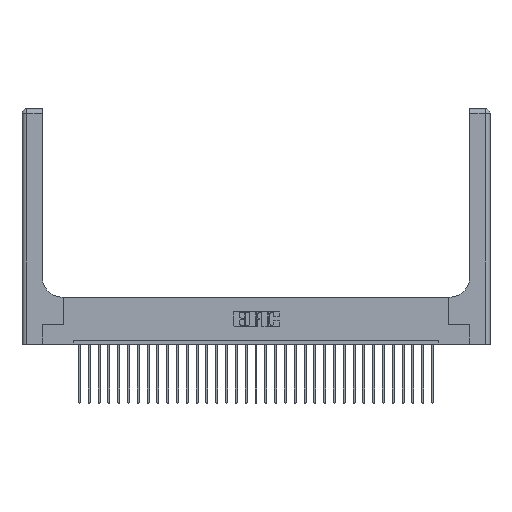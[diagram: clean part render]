
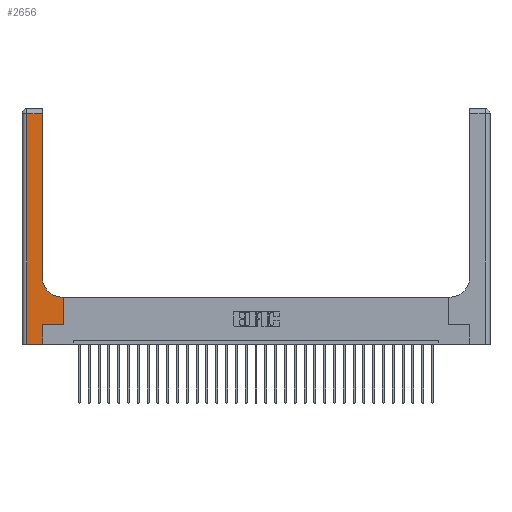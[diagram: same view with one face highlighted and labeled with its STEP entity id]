
A CAD part, top view. The second image highlights one B-rep face of the part: STEP entity #2656.
In plain terms, the highlighted planar face has unit normal (0, 0, 1).
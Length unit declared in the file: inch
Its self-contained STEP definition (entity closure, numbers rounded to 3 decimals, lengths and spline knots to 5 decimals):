
#315 = LINE ( 'NONE', #9708, #10442 ) ;
#465 = LINE ( 'NONE', #26580, #18262 ) ;
#1028 = CARTESIAN_POINT ( 'NONE',  ( 0.06, 2.94, 0.37 ) ) ;
#1530 = VERTEX_POINT ( 'NONE', #1028 ) ;
#1905 = DIRECTION ( 'NONE',  ( 1., 0., 0. ) ) ;
#2060 = AXIS2_PLACEMENT_3D ( 'NONE', #4307, #26555, #17559 ) ;
#2261 = PLANE ( 'NONE',  #2060 ) ;
#2656 = ADVANCED_FACE ( 'NONE', ( #13758 ), #2261, .F. ) ;
#3243 = EDGE_LOOP ( 'NONE', ( #20814, #25991, #20159, #15601, #27370, #13819, #28604, #8238, #14146 ) ) ;
#4156 = CARTESIAN_POINT ( 'NONE',  ( 0.06, 0., 0.37 ) ) ;
#4307 = CARTESIAN_POINT ( 'NONE',  ( 0., 3., 0.37 ) ) ;
#4624 = CARTESIAN_POINT ( 'NONE',  ( 0.26, 0.85, 0.37 ) ) ;
#4829 = CARTESIAN_POINT ( 'NONE',  ( 0.26, 0.6, 0.37 ) ) ;
#5060 = VERTEX_POINT ( 'NONE', #23162 ) ;
#5528 = VERTEX_POINT ( 'NONE', #27013 ) ;
#6109 = CARTESIAN_POINT ( 'NONE',  ( 0.528, 0.25, 0.37 ) ) ;
#6257 = LINE ( 'NONE', #7695, #22923 ) ;
#6574 = EDGE_CURVE ( 'NONE', #18938, #14575, #12671, .T. ) ;
#6727 = DIRECTION ( 'NONE',  ( 0., 0., -1. ) ) ;
#6831 = CARTESIAN_POINT ( 'NONE',  ( 0.51, 0.85, 0.37 ) ) ;
#7682 = CARTESIAN_POINT ( 'NONE',  ( 0.265, 0., 0.37 ) ) ;
#7695 = CARTESIAN_POINT ( 'NONE',  ( 0., 0., 0.37 ) ) ;
#7846 = VERTEX_POINT ( 'NONE', #4624 ) ;
#8238 = ORIENTED_EDGE ( 'NONE', *, *, #27225, .T. ) ;
#8565 = VECTOR ( 'NONE', #14538, 39.37008 ) ;
#9128 = EDGE_CURVE ( 'NONE', #26502, #1530, #315, .T. ) ;
#9708 = CARTESIAN_POINT ( 'NONE',  ( 0., 2.94, 0.37 ) ) ;
#9803 = DIRECTION ( 'NONE',  ( 0., 1., 0. ) ) ;
#10442 = VECTOR ( 'NONE', #12312, 39.37008 ) ;
#10551 = CARTESIAN_POINT ( 'NONE',  ( 0.26, 2.94, 0.37 ) ) ;
#10608 = VECTOR ( 'NONE', #28152, 39.37008 ) ;
#11121 = LINE ( 'NONE', #4829, #25053 ) ;
#11143 = EDGE_CURVE ( 'NONE', #5528, #21543, #12041, .T. ) ;
#11441 = EDGE_CURVE ( 'NONE', #1530, #25163, #14469, .T. ) ;
#11576 = CARTESIAN_POINT ( 'NONE',  ( 0.265, 0.25, 0.37 ) ) ;
#11879 = CIRCLE ( 'NONE', #26289, 0.25 ) ;
#12041 = LINE ( 'NONE', #7682, #13071 ) ;
#12312 = DIRECTION ( 'NONE',  ( -1., 0., 0. ) ) ;
#12671 = LINE ( 'NONE', #6109, #10608 ) ;
#13071 = VECTOR ( 'NONE', #9803, 39.37008 ) ;
#13758 = FACE_OUTER_BOUND ( 'NONE', #3243, .T. ) ;
#13819 = ORIENTED_EDGE ( 'NONE', *, *, #14448, .T. ) ;
#14146 = ORIENTED_EDGE ( 'NONE', *, *, #15593, .T. ) ;
#14448 = EDGE_CURVE ( 'NONE', #21543, #18938, #465, .T. ) ;
#14469 = LINE ( 'NONE', #23480, #8565 ) ;
#14538 = DIRECTION ( 'NONE',  ( 0., -1., 0. ) ) ;
#14575 = VERTEX_POINT ( 'NONE', #28633 ) ;
#15593 = EDGE_CURVE ( 'NONE', #5060, #7846, #11879, .T. ) ;
#15601 = ORIENTED_EDGE ( 'NONE', *, *, #17993, .T. ) ;
#17559 = DIRECTION ( 'NONE',  ( -1., 0., 0. ) ) ;
#17993 = EDGE_CURVE ( 'NONE', #25163, #5528, #6257, .T. ) ;
#18211 = VECTOR ( 'NONE', #27419, 39.37008 ) ;
#18262 = VECTOR ( 'NONE', #1905, 39.37008 ) ;
#18622 = CARTESIAN_POINT ( 'NONE',  ( 0.26, 3., 0.37 ) ) ;
#18938 = VERTEX_POINT ( 'NONE', #27771 ) ;
#20100 = DIRECTION ( 'NONE',  ( -1., 0., 0. ) ) ;
#20159 = ORIENTED_EDGE ( 'NONE', *, *, #11441, .T. ) ;
#20814 = ORIENTED_EDGE ( 'NONE', *, *, #25283, .T. ) ;
#21543 = VERTEX_POINT ( 'NONE', #11576 ) ;
#22923 = VECTOR ( 'NONE', #25561, 39.37008 ) ;
#23162 = CARTESIAN_POINT ( 'NONE',  ( 0.51, 0.6, 0.37 ) ) ;
#23480 = CARTESIAN_POINT ( 'NONE',  ( 0.06, 3., 0.37 ) ) ;
#24098 = LINE ( 'NONE', #18622, #18211 ) ;
#24800 = DIRECTION ( 'NONE',  ( 1., 0., 0. ) ) ;
#25053 = VECTOR ( 'NONE', #20100, 39.37008 ) ;
#25163 = VERTEX_POINT ( 'NONE', #4156 ) ;
#25283 = EDGE_CURVE ( 'NONE', #7846, #26502, #24098, .T. ) ;
#25561 = DIRECTION ( 'NONE',  ( 1., 0., 0. ) ) ;
#25991 = ORIENTED_EDGE ( 'NONE', *, *, #9128, .T. ) ;
#26289 = AXIS2_PLACEMENT_3D ( 'NONE', #6831, #6727, #24800 ) ;
#26502 = VERTEX_POINT ( 'NONE', #10551 ) ;
#26555 = DIRECTION ( 'NONE',  ( 0., 0., -1. ) ) ;
#26580 = CARTESIAN_POINT ( 'NONE',  ( 0.265, 0.25, 0.37 ) ) ;
#27013 = CARTESIAN_POINT ( 'NONE',  ( 0.265, 0., 0.37 ) ) ;
#27225 = EDGE_CURVE ( 'NONE', #14575, #5060, #11121, .T. ) ;
#27370 = ORIENTED_EDGE ( 'NONE', *, *, #11143, .T. ) ;
#27419 = DIRECTION ( 'NONE',  ( 0., 1., 0. ) ) ;
#27771 = CARTESIAN_POINT ( 'NONE',  ( 0.528, 0.25, 0.37 ) ) ;
#28152 = DIRECTION ( 'NONE',  ( 0., 1., 0. ) ) ;
#28604 = ORIENTED_EDGE ( 'NONE', *, *, #6574, .T. ) ;
#28633 = CARTESIAN_POINT ( 'NONE',  ( 0.528, 0.6, 0.37 ) ) ;
